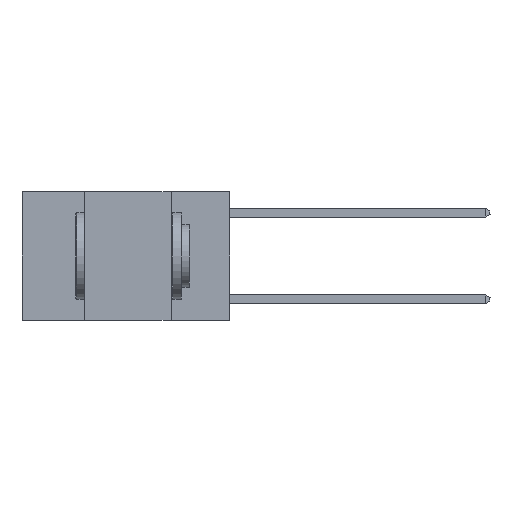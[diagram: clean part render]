
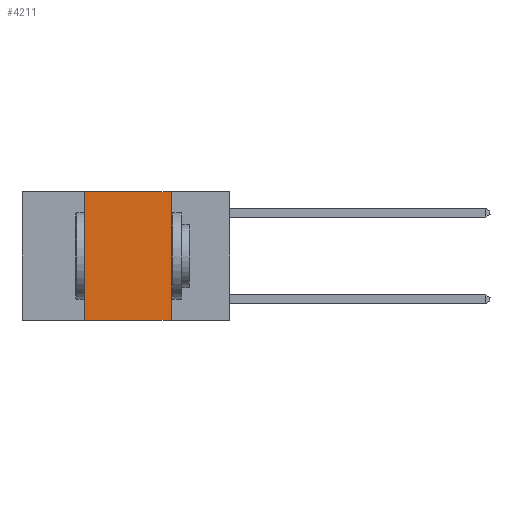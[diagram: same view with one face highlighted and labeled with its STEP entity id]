
A CAD part, left-side view. The second image highlights one B-rep face of the part: STEP entity #4211.
In plain terms, the highlighted planar face has unit normal (-1, 0, 0).
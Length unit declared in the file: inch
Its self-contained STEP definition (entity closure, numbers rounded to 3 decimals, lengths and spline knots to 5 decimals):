
#52 = DIRECTION ( 'NONE',  ( 1., 0., 0. ) ) ;
#1653 = CARTESIAN_POINT ( 'NONE',  ( 0., 0.6, 0. ) ) ;
#1818 = CARTESIAN_POINT ( 'NONE',  ( 0., 0.6, -0.37 ) ) ;
#2451 = VERTEX_POINT ( 'NONE', #5137 ) ;
#2526 = ORIENTED_EDGE ( 'NONE', *, *, #12685, .F. ) ;
#2538 = PLANE ( 'NONE',  #5596 ) ;
#2785 = EDGE_CURVE ( 'NONE', #6242, #15582, #3941, .T. ) ;
#3941 = LINE ( 'NONE', #14814, #7571 ) ;
#4211 = ADVANCED_FACE ( 'NONE', ( #5943 ), #2538, .F. ) ;
#4496 = DIRECTION ( 'NONE',  ( 0., -1., 0. ) ) ;
#4889 = ORIENTED_EDGE ( 'NONE', *, *, #11331, .F. ) ;
#5036 = VECTOR ( 'NONE', #7747, 39.37008 ) ;
#5086 = VECTOR ( 'NONE', #4496, 39.37008 ) ;
#5137 = CARTESIAN_POINT ( 'NONE',  ( 0., 0.42, 0. ) ) ;
#5596 = AXIS2_PLACEMENT_3D ( 'NONE', #9605, #52, #6088 ) ;
#5943 = FACE_OUTER_BOUND ( 'NONE', #6231, .T. ) ;
#6074 = VECTOR ( 'NONE', #14941, 39.37008 ) ;
#6088 = DIRECTION ( 'NONE',  ( 0., 0., -1. ) ) ;
#6231 = EDGE_LOOP ( 'NONE', ( #8903, #4889, #2526, #11462 ) ) ;
#6242 = VERTEX_POINT ( 'NONE', #14084 ) ;
#7571 = VECTOR ( 'NONE', #7807, 39.37008 ) ;
#7747 = DIRECTION ( 'NONE',  ( 0., -1., 0. ) ) ;
#7807 = DIRECTION ( 'NONE',  ( 0., 0., -1. ) ) ;
#8903 = ORIENTED_EDGE ( 'NONE', *, *, #2785, .F. ) ;
#9139 = CARTESIAN_POINT ( 'NONE',  ( 0., 0.42, 0. ) ) ;
#9439 = LINE ( 'NONE', #1818, #5086 ) ;
#9605 = CARTESIAN_POINT ( 'NONE',  ( 0., 0.6, 0. ) ) ;
#9723 = EDGE_CURVE ( 'NONE', #11227, #15582, #9439, .T. ) ;
#11227 = VERTEX_POINT ( 'NONE', #12349 ) ;
#11331 = EDGE_CURVE ( 'NONE', #2451, #6242, #12658, .T. ) ;
#11462 = ORIENTED_EDGE ( 'NONE', *, *, #9723, .T. ) ;
#12349 = CARTESIAN_POINT ( 'NONE',  ( 0., 0.42, -0.37 ) ) ;
#12658 = LINE ( 'NONE', #1653, #5036 ) ;
#12685 = EDGE_CURVE ( 'NONE', #11227, #2451, #15170, .T. ) ;
#14084 = CARTESIAN_POINT ( 'NONE',  ( 0., 0.17, 0. ) ) ;
#14814 = CARTESIAN_POINT ( 'NONE',  ( 0., 0.17, 0. ) ) ;
#14941 = DIRECTION ( 'NONE',  ( 0., 0., 1. ) ) ;
#15170 = LINE ( 'NONE', #9139, #6074 ) ;
#15519 = CARTESIAN_POINT ( 'NONE',  ( 0., 0.17, -0.37 ) ) ;
#15582 = VERTEX_POINT ( 'NONE', #15519 ) ;
